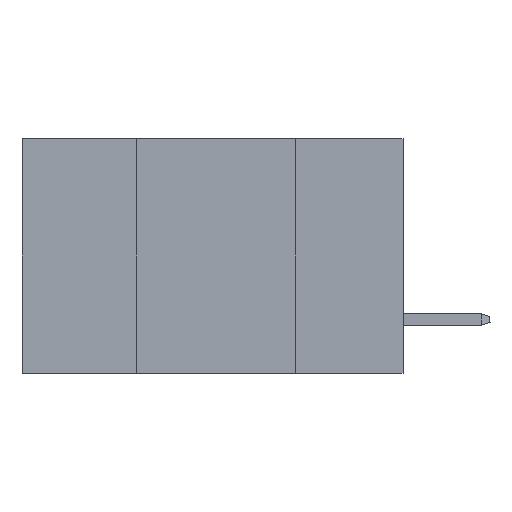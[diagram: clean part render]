
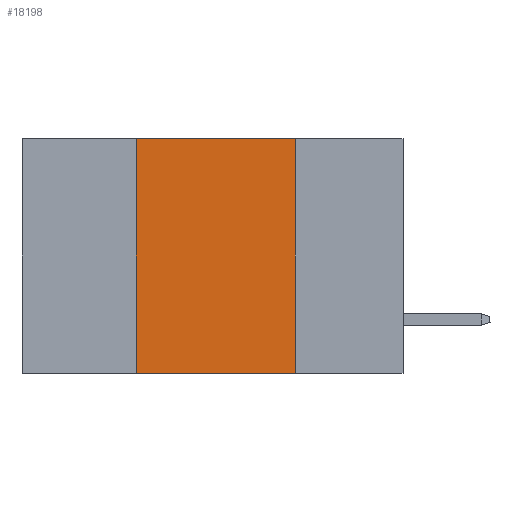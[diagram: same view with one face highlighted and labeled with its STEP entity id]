
A CAD part, left-side view. The second image highlights one B-rep face of the part: STEP entity #18198.
In plain terms, the highlighted planar face has unit normal (-1, 0, 0).
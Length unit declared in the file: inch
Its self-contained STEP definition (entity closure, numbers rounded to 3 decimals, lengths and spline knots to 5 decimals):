
#1296 = CARTESIAN_POINT ( 'NONE',  ( 0., 0.6, -0.37 ) ) ;
#3345 = CARTESIAN_POINT ( 'NONE',  ( 0., 0.17, 0. ) ) ;
#4165 = FACE_OUTER_BOUND ( 'NONE', #14281, .T. ) ;
#4791 = DIRECTION ( 'NONE',  ( 0., -1., 0. ) ) ;
#7292 = ORIENTED_EDGE ( 'NONE', *, *, #22453, .F. ) ;
#7941 = VECTOR ( 'NONE', #37442, 39.37008 ) ;
#8857 = VECTOR ( 'NONE', #4791, 39.37008 ) ;
#9273 = ORIENTED_EDGE ( 'NONE', *, *, #22695, .T. ) ;
#13004 = CARTESIAN_POINT ( 'NONE',  ( 0., 0.42, 0. ) ) ;
#13233 = CARTESIAN_POINT ( 'NONE',  ( 0., 0.6, 0. ) ) ;
#14281 = EDGE_LOOP ( 'NONE', ( #7292, #25264, #26883, #9273 ) ) ;
#14827 = LINE ( 'NONE', #17766, #38182 ) ;
#15115 = VECTOR ( 'NONE', #36345, 39.37008 ) ;
#15738 = DIRECTION ( 'NONE',  ( 1., 0., 0. ) ) ;
#16136 = CARTESIAN_POINT ( 'NONE',  ( 0., 0.6, 0. ) ) ;
#16439 = VERTEX_POINT ( 'NONE', #25758 ) ;
#17766 = CARTESIAN_POINT ( 'NONE',  ( 0., 0.17, 0. ) ) ;
#18116 = CARTESIAN_POINT ( 'NONE',  ( 0., 0.42, -0.37 ) ) ;
#18198 = ADVANCED_FACE ( 'NONE', ( #4165 ), #30979, .F. ) ;
#21786 = DIRECTION ( 'NONE',  ( 0., 0., -1. ) ) ;
#22453 = EDGE_CURVE ( 'NONE', #28726, #16439, #14827, .T. ) ;
#22695 = EDGE_CURVE ( 'NONE', #29590, #16439, #31597, .T. ) ;
#25264 = ORIENTED_EDGE ( 'NONE', *, *, #34624, .F. ) ;
#25758 = CARTESIAN_POINT ( 'NONE',  ( 0., 0.17, -0.37 ) ) ;
#26338 = EDGE_CURVE ( 'NONE', #29590, #28444, #35974, .T. ) ;
#26587 = CARTESIAN_POINT ( 'NONE',  ( 0., 0.42, 0. ) ) ;
#26883 = ORIENTED_EDGE ( 'NONE', *, *, #26338, .F. ) ;
#28444 = VERTEX_POINT ( 'NONE', #13004 ) ;
#28726 = VERTEX_POINT ( 'NONE', #3345 ) ;
#29590 = VERTEX_POINT ( 'NONE', #18116 ) ;
#30631 = LINE ( 'NONE', #13233, #7941 ) ;
#30979 = PLANE ( 'NONE',  #37710 ) ;
#31597 = LINE ( 'NONE', #1296, #8857 ) ;
#32791 = DIRECTION ( 'NONE',  ( 0., 0., -1. ) ) ;
#34624 = EDGE_CURVE ( 'NONE', #28444, #28726, #30631, .T. ) ;
#35974 = LINE ( 'NONE', #26587, #15115 ) ;
#36345 = DIRECTION ( 'NONE',  ( 0., 0., 1. ) ) ;
#37442 = DIRECTION ( 'NONE',  ( 0., -1., 0. ) ) ;
#37710 = AXIS2_PLACEMENT_3D ( 'NONE', #16136, #15738, #21786 ) ;
#38182 = VECTOR ( 'NONE', #32791, 39.37008 ) ;
